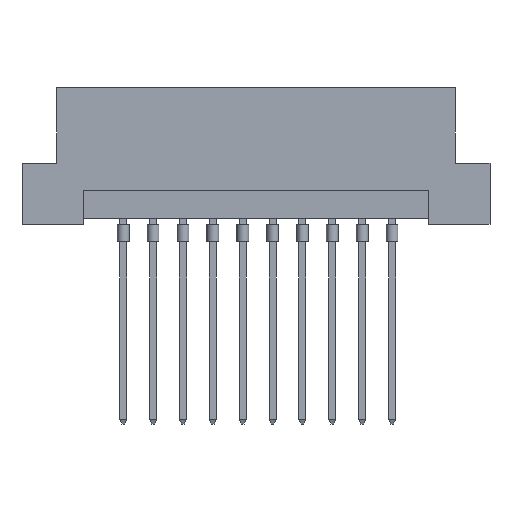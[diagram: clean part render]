
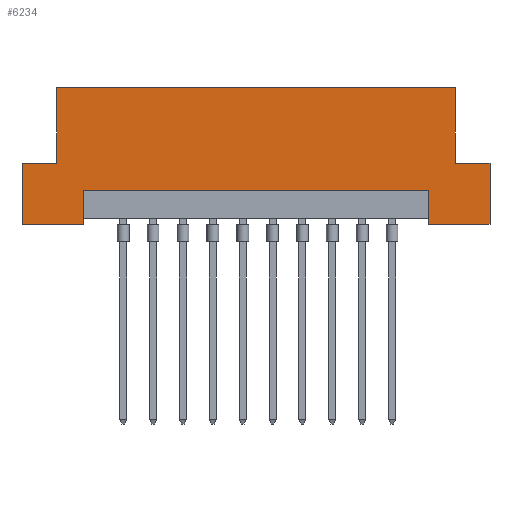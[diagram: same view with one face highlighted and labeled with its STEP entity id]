
A CAD part, front view. The second image highlights one B-rep face of the part: STEP entity #6234.
In plain terms, the highlighted planar face has unit normal (0, -1, 0).
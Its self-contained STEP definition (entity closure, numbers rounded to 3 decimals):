
#110 = LINE ( 'NONE', #4550, #3918 ) ;
#258 = EDGE_CURVE ( 'NONE', #1085, #6933, #5091, .T. ) ;
#302 = VERTEX_POINT ( 'NONE', #6850 ) ;
#503 = CARTESIAN_POINT ( 'NONE',  ( -19.9, 0., 0. ) ) ;
#627 = VERTEX_POINT ( 'NONE', #1083 ) ;
#647 = VECTOR ( 'NONE', #3444, 1000. ) ;
#746 = ORIENTED_EDGE ( 'NONE', *, *, #6036, .T. ) ;
#810 = CARTESIAN_POINT ( 'NONE',  ( -14.69, 0., 2.9 ) ) ;
#883 = LINE ( 'NONE', #4767, #6261 ) ;
#987 = CARTESIAN_POINT ( 'NONE',  ( -19.9, 0., 5.2 ) ) ;
#1083 = CARTESIAN_POINT ( 'NONE',  ( -19.9, 0., 0. ) ) ;
#1085 = VERTEX_POINT ( 'NONE', #6012 ) ;
#1164 = LINE ( 'NONE', #5559, #4467 ) ;
#1186 = VERTEX_POINT ( 'NONE', #4176 ) ;
#1210 = CARTESIAN_POINT ( 'NONE',  ( 19.9, 0., 5.2 ) ) ;
#1240 = VECTOR ( 'NONE', #4527, 1000. ) ;
#1329 = LINE ( 'NONE', #6749, #4379 ) ;
#1603 = CARTESIAN_POINT ( 'NONE',  ( -19.9, 0., 11.6 ) ) ;
#1606 = VERTEX_POINT ( 'NONE', #1210 ) ;
#1616 = EDGE_CURVE ( 'NONE', #6287, #5574, #6779, .T. ) ;
#1625 = CARTESIAN_POINT ( 'NONE',  ( -14.69, 0., 0. ) ) ;
#1681 = VECTOR ( 'NONE', #3837, 1000. ) ;
#2018 = LINE ( 'NONE', #6505, #6500 ) ;
#2021 = EDGE_CURVE ( 'NONE', #302, #6727, #5590, .T. ) ;
#2037 = DIRECTION ( 'NONE',  ( 0., 0., -1. ) ) ;
#2329 = CARTESIAN_POINT ( 'NONE',  ( 14.69, 0., 2.9 ) ) ;
#2344 = VERTEX_POINT ( 'NONE', #3142 ) ;
#2432 = ORIENTED_EDGE ( 'NONE', *, *, #3491, .F. ) ;
#2496 = ORIENTED_EDGE ( 'NONE', *, *, #3207, .F. ) ;
#2597 = FACE_OUTER_BOUND ( 'NONE', #4714, .T. ) ;
#2621 = VECTOR ( 'NONE', #3999, 1000. ) ;
#2742 = CARTESIAN_POINT ( 'NONE',  ( -16.94, 0., 5.2 ) ) ;
#2851 = CARTESIAN_POINT ( 'NONE',  ( 19.9, 0., 5.2 ) ) ;
#2936 = ORIENTED_EDGE ( 'NONE', *, *, #5042, .T. ) ;
#3103 = EDGE_CURVE ( 'NONE', #6727, #4700, #110, .T. ) ;
#3142 = CARTESIAN_POINT ( 'NONE',  ( 16.94, 0., 5.2 ) ) ;
#3207 = EDGE_CURVE ( 'NONE', #6775, #627, #1329, .T. ) ;
#3283 = CARTESIAN_POINT ( 'NONE',  ( -14.69, 0., 0.5 ) ) ;
#3299 = EDGE_CURVE ( 'NONE', #1606, #6287, #883, .T. ) ;
#3360 = DIRECTION ( 'NONE',  ( 0., 0., -1. ) ) ;
#3384 = ORIENTED_EDGE ( 'NONE', *, *, #3299, .F. ) ;
#3386 = CARTESIAN_POINT ( 'NONE',  ( 16.94, 0., 5.2 ) ) ;
#3444 = DIRECTION ( 'NONE',  ( -1., 0., 0. ) ) ;
#3458 = DIRECTION ( 'NONE',  ( 1., 0., 0. ) ) ;
#3491 = EDGE_CURVE ( 'NONE', #1186, #302, #5998, .T. ) ;
#3532 = ORIENTED_EDGE ( 'NONE', *, *, #2021, .F. ) ;
#3579 = VECTOR ( 'NONE', #3839, 1000. ) ;
#3766 = PLANE ( 'NONE',  #4120 ) ;
#3811 = LINE ( 'NONE', #3283, #3579 ) ;
#3833 = LINE ( 'NONE', #2851, #1240 ) ;
#3837 = DIRECTION ( 'NONE',  ( 0., 0., 1. ) ) ;
#3839 = DIRECTION ( 'NONE',  ( 0., 0., -1. ) ) ;
#3887 = EDGE_CURVE ( 'NONE', #2344, #1606, #3833, .T. ) ;
#3918 = VECTOR ( 'NONE', #3458, 1000. ) ;
#3999 = DIRECTION ( 'NONE',  ( -1., 0., 0. ) ) ;
#4120 = AXIS2_PLACEMENT_3D ( 'NONE', #1603, #7153, #6507 ) ;
#4176 = CARTESIAN_POINT ( 'NONE',  ( -19.9, 0., 5.2 ) ) ;
#4229 = CARTESIAN_POINT ( 'NONE',  ( 19.9, 0., 0. ) ) ;
#4379 = VECTOR ( 'NONE', #5213, 1000. ) ;
#4425 = EDGE_CURVE ( 'NONE', #6933, #6775, #3811, .T. ) ;
#4467 = VECTOR ( 'NONE', #3360, 1000. ) ;
#4515 = CARTESIAN_POINT ( 'NONE',  ( 14.69, 0., 0. ) ) ;
#4527 = DIRECTION ( 'NONE',  ( 1., 0., 0. ) ) ;
#4550 = CARTESIAN_POINT ( 'NONE',  ( -19.9, 0., 11.6 ) ) ;
#4551 = CARTESIAN_POINT ( 'NONE',  ( -16.94, 0., 11.6 ) ) ;
#4700 = VERTEX_POINT ( 'NONE', #6296 ) ;
#4714 = EDGE_LOOP ( 'NONE', ( #6921, #746, #6780, #3384, #5739, #2936, #6450, #3532, #2432, #4807, #2496, #6156 ) ) ;
#4767 = CARTESIAN_POINT ( 'NONE',  ( 19.9, 0., 0. ) ) ;
#4807 = ORIENTED_EDGE ( 'NONE', *, *, #5015, .F. ) ;
#5015 = EDGE_CURVE ( 'NONE', #627, #1186, #2018, .T. ) ;
#5042 = EDGE_CURVE ( 'NONE', #2344, #4700, #7151, .T. ) ;
#5091 = LINE ( 'NONE', #2329, #2621 ) ;
#5213 = DIRECTION ( 'NONE',  ( -1., 0., 0. ) ) ;
#5327 = VECTOR ( 'NONE', #5461, 1000. ) ;
#5461 = DIRECTION ( 'NONE',  ( 1., 0., 0. ) ) ;
#5559 = CARTESIAN_POINT ( 'NONE',  ( 14.69, 0., 0.5 ) ) ;
#5574 = VERTEX_POINT ( 'NONE', #4515 ) ;
#5590 = LINE ( 'NONE', #2742, #1681 ) ;
#5739 = ORIENTED_EDGE ( 'NONE', *, *, #3887, .F. ) ;
#5998 = LINE ( 'NONE', #987, #5327 ) ;
#6012 = CARTESIAN_POINT ( 'NONE',  ( 14.69, 0., 2.9 ) ) ;
#6036 = EDGE_CURVE ( 'NONE', #1085, #5574, #1164, .T. ) ;
#6156 = ORIENTED_EDGE ( 'NONE', *, *, #4425, .F. ) ;
#6208 = DIRECTION ( 'NONE',  ( 0., 0., 1. ) ) ;
#6234 = ADVANCED_FACE ( 'NONE', ( #2597 ), #3766, .F. ) ;
#6261 = VECTOR ( 'NONE', #2037, 1000. ) ;
#6287 = VERTEX_POINT ( 'NONE', #4229 ) ;
#6296 = CARTESIAN_POINT ( 'NONE',  ( 16.94, 0., 11.6 ) ) ;
#6450 = ORIENTED_EDGE ( 'NONE', *, *, #3103, .F. ) ;
#6500 = VECTOR ( 'NONE', #6577, 1000. ) ;
#6505 = CARTESIAN_POINT ( 'NONE',  ( -19.9, 0., 0. ) ) ;
#6507 = DIRECTION ( 'NONE',  ( 0., 0., 1. ) ) ;
#6577 = DIRECTION ( 'NONE',  ( 0., 0., 1. ) ) ;
#6622 = VECTOR ( 'NONE', #6208, 1000. ) ;
#6727 = VERTEX_POINT ( 'NONE', #4551 ) ;
#6749 = CARTESIAN_POINT ( 'NONE',  ( -19.9, 0., 0. ) ) ;
#6775 = VERTEX_POINT ( 'NONE', #1625 ) ;
#6779 = LINE ( 'NONE', #503, #647 ) ;
#6780 = ORIENTED_EDGE ( 'NONE', *, *, #1616, .F. ) ;
#6850 = CARTESIAN_POINT ( 'NONE',  ( -16.94, 0., 5.2 ) ) ;
#6921 = ORIENTED_EDGE ( 'NONE', *, *, #258, .F. ) ;
#6933 = VERTEX_POINT ( 'NONE', #810 ) ;
#7151 = LINE ( 'NONE', #3386, #6622 ) ;
#7153 = DIRECTION ( 'NONE',  ( 0., 1., 0. ) ) ;
